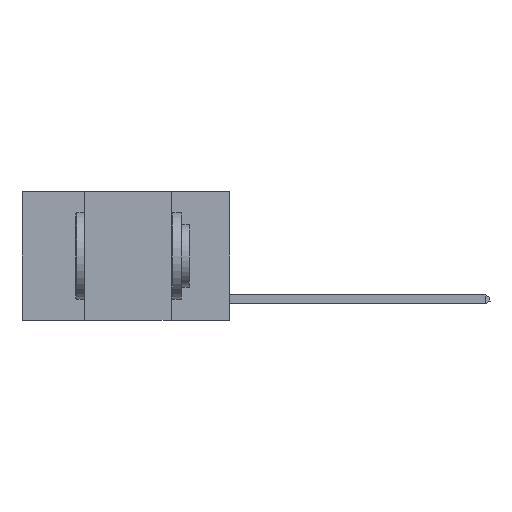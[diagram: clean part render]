
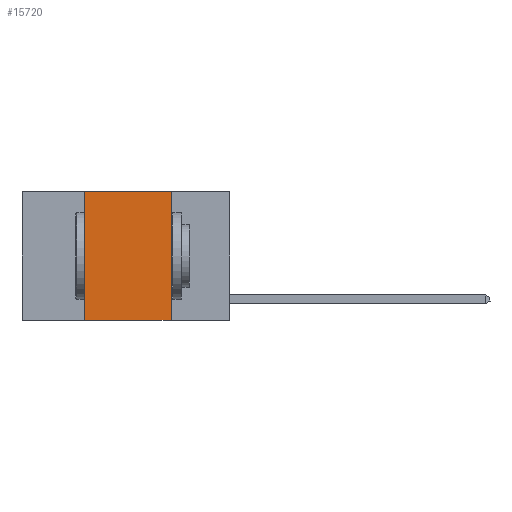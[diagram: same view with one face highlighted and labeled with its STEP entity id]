
A CAD part, left-side view. The second image highlights one B-rep face of the part: STEP entity #15720.
In plain terms, the highlighted planar face has unit normal (-1, 0, 0).
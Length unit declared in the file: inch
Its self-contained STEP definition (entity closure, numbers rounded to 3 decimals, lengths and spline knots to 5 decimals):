
#116 = VECTOR ( 'NONE', #12226, 39.37008 ) ;
#381 = CARTESIAN_POINT ( 'NONE',  ( 0., 0.42, -0.37 ) ) ;
#448 = CARTESIAN_POINT ( 'NONE',  ( 0., 0.42, 0. ) ) ;
#471 = CARTESIAN_POINT ( 'NONE',  ( 0., 0.6, 0. ) ) ;
#921 = VERTEX_POINT ( 'NONE', #17791 ) ;
#1649 = VECTOR ( 'NONE', #16040, 39.37008 ) ;
#2779 = VERTEX_POINT ( 'NONE', #381 ) ;
#2901 = EDGE_CURVE ( 'NONE', #2779, #26448, #14522, .T. ) ;
#3227 = ORIENTED_EDGE ( 'NONE', *, *, #4472, .F. ) ;
#3842 = CARTESIAN_POINT ( 'NONE',  ( 0., 0.42, 0. ) ) ;
#4430 = LINE ( 'NONE', #6415, #22420 ) ;
#4472 = EDGE_CURVE ( 'NONE', #921, #26448, #22649, .T. ) ;
#5914 = ORIENTED_EDGE ( 'NONE', *, *, #14760, .F. ) ;
#6415 = CARTESIAN_POINT ( 'NONE',  ( 0., 0.6, 0. ) ) ;
#7074 = EDGE_CURVE ( 'NONE', #2779, #19577, #14056, .T. ) ;
#9163 = DIRECTION ( 'NONE',  ( 1., 0., 0. ) ) ;
#11230 = ORIENTED_EDGE ( 'NONE', *, *, #7074, .F. ) ;
#11333 = FACE_OUTER_BOUND ( 'NONE', #23961, .T. ) ;
#12226 = DIRECTION ( 'NONE',  ( 0., -1., 0. ) ) ;
#12361 = CARTESIAN_POINT ( 'NONE',  ( 0., 0.6, -0.37 ) ) ;
#12654 = CARTESIAN_POINT ( 'NONE',  ( 0., 0.17, -0.37 ) ) ;
#14056 = LINE ( 'NONE', #448, #1649 ) ;
#14522 = LINE ( 'NONE', #12361, #116 ) ;
#14760 = EDGE_CURVE ( 'NONE', #19577, #921, #4430, .T. ) ;
#15361 = PLANE ( 'NONE',  #15603 ) ;
#15603 = AXIS2_PLACEMENT_3D ( 'NONE', #471, #9163, #17910 ) ;
#15720 = ADVANCED_FACE ( 'NONE', ( #11333 ), #15361, .F. ) ;
#16040 = DIRECTION ( 'NONE',  ( 0., 0., 1. ) ) ;
#16729 = ORIENTED_EDGE ( 'NONE', *, *, #2901, .T. ) ;
#17791 = CARTESIAN_POINT ( 'NONE',  ( 0., 0.17, 0. ) ) ;
#17910 = DIRECTION ( 'NONE',  ( 0., 0., -1. ) ) ;
#19577 = VERTEX_POINT ( 'NONE', #3842 ) ;
#20500 = DIRECTION ( 'NONE',  ( 0., 0., -1. ) ) ;
#22420 = VECTOR ( 'NONE', #23763, 39.37008 ) ;
#22649 = LINE ( 'NONE', #26511, #26877 ) ;
#23763 = DIRECTION ( 'NONE',  ( 0., -1., 0. ) ) ;
#23961 = EDGE_LOOP ( 'NONE', ( #3227, #5914, #11230, #16729 ) ) ;
#26448 = VERTEX_POINT ( 'NONE', #12654 ) ;
#26511 = CARTESIAN_POINT ( 'NONE',  ( 0., 0.17, 0. ) ) ;
#26877 = VECTOR ( 'NONE', #20500, 39.37008 ) ;
